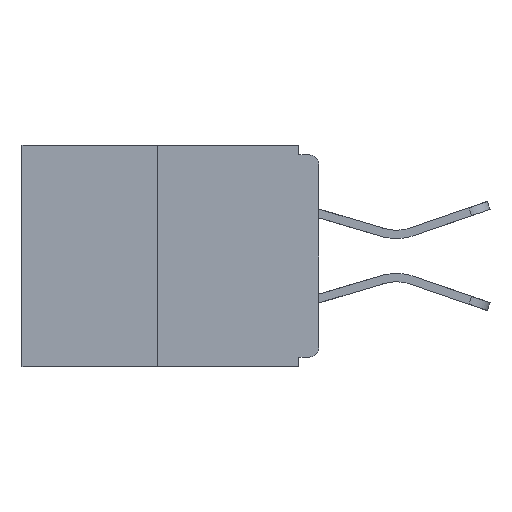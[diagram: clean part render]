
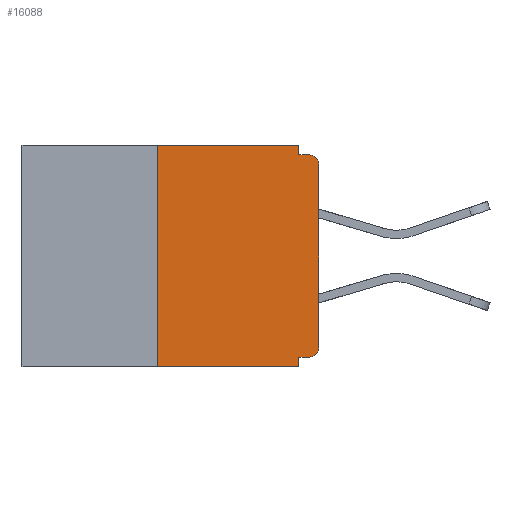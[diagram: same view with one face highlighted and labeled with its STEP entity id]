
A CAD part, left-side view. The second image highlights one B-rep face of the part: STEP entity #16088.
In plain terms, the highlighted planar face has unit normal (-1, 0, 0).
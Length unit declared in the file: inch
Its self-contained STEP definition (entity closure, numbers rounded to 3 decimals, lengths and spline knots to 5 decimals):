
#36 = VERTEX_POINT ( 'NONE', #16436 ) ;
#232 = EDGE_CURVE ( 'NONE', #5543, #1355, #12804, .T. ) ;
#381 = ORIENTED_EDGE ( 'NONE', *, *, #21592, .F. ) ;
#767 = VERTEX_POINT ( 'NONE', #2600 ) ;
#806 = CARTESIAN_POINT ( 'NONE',  ( 0., 0., -0.03 ) ) ;
#845 = LINE ( 'NONE', #24581, #24061 ) ;
#1155 = CARTESIAN_POINT ( 'NONE',  ( 0., 0.031, -0.015 ) ) ;
#1309 = CARTESIAN_POINT ( 'NONE',  ( 0., 0.25, 0. ) ) ;
#1353 = VECTOR ( 'NONE', #22451, 39.37008 ) ;
#1355 = VERTEX_POINT ( 'NONE', #18018 ) ;
#1434 = LINE ( 'NONE', #15354, #7051 ) ;
#2600 = CARTESIAN_POINT ( 'NONE',  ( 0., 0.031, -0.328 ) ) ;
#3520 = DIRECTION ( 'NONE',  ( -1., 0., 0. ) ) ;
#4650 = DIRECTION ( 'NONE',  ( 0., 1., 0. ) ) ;
#5014 = DIRECTION ( 'NONE',  ( 0., 0., -1. ) ) ;
#5485 = VERTEX_POINT ( 'NONE', #806 ) ;
#5543 = VERTEX_POINT ( 'NONE', #1155 ) ;
#5789 = DIRECTION ( 'NONE',  ( 0., -1., 0. ) ) ;
#6306 = ORIENTED_EDGE ( 'NONE', *, *, #22135, .F. ) ;
#6646 = ORIENTED_EDGE ( 'NONE', *, *, #232, .F. ) ;
#6893 = CARTESIAN_POINT ( 'NONE',  ( 0., 0.015, -0.03 ) ) ;
#7018 = ORIENTED_EDGE ( 'NONE', *, *, #11525, .F. ) ;
#7051 = VECTOR ( 'NONE', #4650, 39.37008 ) ;
#7126 = VERTEX_POINT ( 'NONE', #15013 ) ;
#7265 = ORIENTED_EDGE ( 'NONE', *, *, #16677, .T. ) ;
#7599 = ORIENTED_EDGE ( 'NONE', *, *, #20931, .F. ) ;
#7611 = CARTESIAN_POINT ( 'NONE',  ( 0., 0.031, -0.343 ) ) ;
#8062 = VERTEX_POINT ( 'NONE', #21007 ) ;
#8248 = CARTESIAN_POINT ( 'NONE',  ( 0., 0.25, 0. ) ) ;
#8378 = CIRCLE ( 'NONE', #18860, 0.015 ) ;
#8462 = LINE ( 'NONE', #10376, #14341 ) ;
#9551 = DIRECTION ( 'NONE',  ( 0., 0., -1. ) ) ;
#9685 = CARTESIAN_POINT ( 'NONE',  ( 0., 0.015, -0.313 ) ) ;
#9980 = EDGE_CURVE ( 'NONE', #5485, #1355, #8378, .T. ) ;
#10376 = CARTESIAN_POINT ( 'NONE',  ( 0., 0.46, -0.343 ) ) ;
#10923 = AXIS2_PLACEMENT_3D ( 'NONE', #17709, #19801, #5014 ) ;
#11525 = EDGE_CURVE ( 'NONE', #767, #26721, #15198, .T. ) ;
#11877 = ORIENTED_EDGE ( 'NONE', *, *, #9980, .T. ) ;
#11944 = CARTESIAN_POINT ( 'NONE',  ( 0., 0., -0.015 ) ) ;
#12082 = VERTEX_POINT ( 'NONE', #8248 ) ;
#12473 = EDGE_CURVE ( 'NONE', #36, #12082, #16116, .T. ) ;
#12804 = LINE ( 'NONE', #11944, #23259 ) ;
#13493 = LINE ( 'NONE', #22792, #22987 ) ;
#13834 = ORIENTED_EDGE ( 'NONE', *, *, #25115, .T. ) ;
#14341 = VECTOR ( 'NONE', #16390, 39.37008 ) ;
#15013 = CARTESIAN_POINT ( 'NONE',  ( 0., 0.015, -0.328 ) ) ;
#15198 = LINE ( 'NONE', #19837, #23698 ) ;
#15354 = CARTESIAN_POINT ( 'NONE',  ( 0., 0., -0.328 ) ) ;
#16088 = ADVANCED_FACE ( 'NONE', ( #17352 ), #18449, .F. ) ;
#16116 = LINE ( 'NONE', #1309, #1353 ) ;
#16390 = DIRECTION ( 'NONE',  ( 0., -1., 0. ) ) ;
#16436 = CARTESIAN_POINT ( 'NONE',  ( 0., 0.25, -0.343 ) ) ;
#16677 = EDGE_CURVE ( 'NONE', #7126, #8062, #17948, .T. ) ;
#16934 = ORIENTED_EDGE ( 'NONE', *, *, #21899, .T. ) ;
#17210 = CARTESIAN_POINT ( 'NONE',  ( 0., 0.031, 0. ) ) ;
#17352 = FACE_OUTER_BOUND ( 'NONE', #25570, .T. ) ;
#17651 = DIRECTION ( 'NONE',  ( 0., 0., -1. ) ) ;
#17709 = CARTESIAN_POINT ( 'NONE',  ( 0., 0.46, 0. ) ) ;
#17948 = CIRCLE ( 'NONE', #20875, 0.015 ) ;
#18018 = CARTESIAN_POINT ( 'NONE',  ( 0., 0.015, -0.015 ) ) ;
#18449 = PLANE ( 'NONE',  #10923 ) ;
#18731 = ORIENTED_EDGE ( 'NONE', *, *, #12473, .F. ) ;
#18860 = AXIS2_PLACEMENT_3D ( 'NONE', #6893, #19392, #23885 ) ;
#19392 = DIRECTION ( 'NONE',  ( -1., 0., 0. ) ) ;
#19801 = DIRECTION ( 'NONE',  ( 1., 0., 0. ) ) ;
#19837 = CARTESIAN_POINT ( 'NONE',  ( 0., 0.031, -0.343 ) ) ;
#20153 = DIRECTION ( 'NONE',  ( 0., 0., -1. ) ) ;
#20533 = DIRECTION ( 'NONE',  ( 0., 0., 1. ) ) ;
#20875 = AXIS2_PLACEMENT_3D ( 'NONE', #9685, #3520, #20153 ) ;
#20931 = EDGE_CURVE ( 'NONE', #12082, #21796, #13493, .T. ) ;
#21007 = CARTESIAN_POINT ( 'NONE',  ( 0., 0., -0.313 ) ) ;
#21592 = EDGE_CURVE ( 'NONE', #21796, #5543, #26376, .T. ) ;
#21796 = VERTEX_POINT ( 'NONE', #17210 ) ;
#21899 = EDGE_CURVE ( 'NONE', #8062, #5485, #845, .T. ) ;
#22135 = EDGE_CURVE ( 'NONE', #7126, #767, #1434, .T. ) ;
#22451 = DIRECTION ( 'NONE',  ( 0., 0., 1. ) ) ;
#22792 = CARTESIAN_POINT ( 'NONE',  ( 0., 0.46, 0. ) ) ;
#22987 = VECTOR ( 'NONE', #24515, 39.37008 ) ;
#23259 = VECTOR ( 'NONE', #5789, 39.37008 ) ;
#23698 = VECTOR ( 'NONE', #17651, 39.37008 ) ;
#23885 = DIRECTION ( 'NONE',  ( 0., 0., -1. ) ) ;
#24061 = VECTOR ( 'NONE', #20533, 39.37008 ) ;
#24515 = DIRECTION ( 'NONE',  ( 0., -1., 0. ) ) ;
#24581 = CARTESIAN_POINT ( 'NONE',  ( 0., 0., 0. ) ) ;
#25099 = VECTOR ( 'NONE', #9551, 39.37008 ) ;
#25115 = EDGE_CURVE ( 'NONE', #36, #26721, #8462, .T. ) ;
#25570 = EDGE_LOOP ( 'NONE', ( #7599, #18731, #13834, #7018, #6306, #7265, #16934, #11877, #6646, #381 ) ) ;
#26360 = CARTESIAN_POINT ( 'NONE',  ( 0., 0.031, 0. ) ) ;
#26376 = LINE ( 'NONE', #26360, #25099 ) ;
#26721 = VERTEX_POINT ( 'NONE', #7611 ) ;
